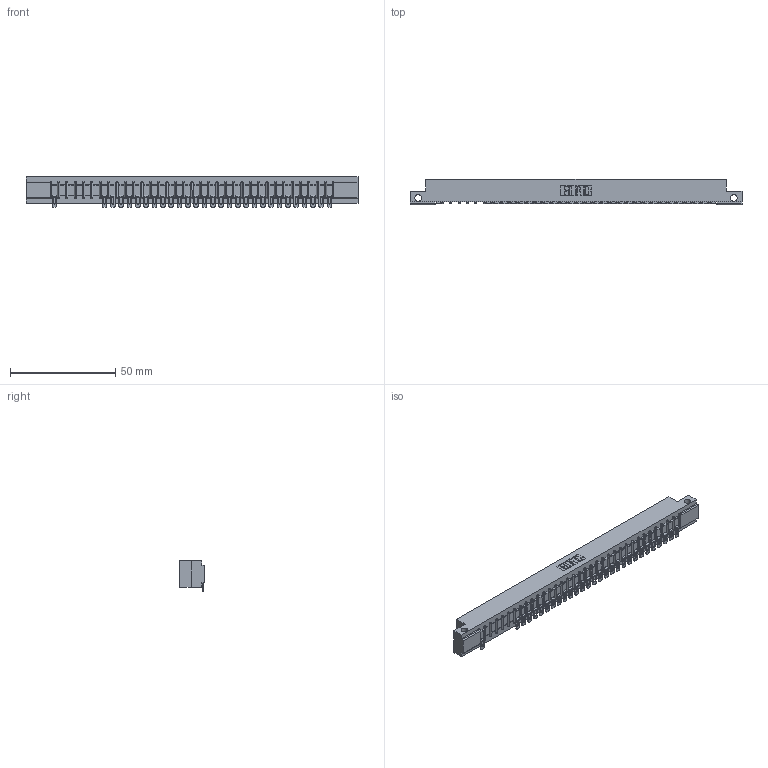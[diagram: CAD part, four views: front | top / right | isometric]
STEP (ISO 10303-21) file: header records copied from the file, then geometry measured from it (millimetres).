
FILE_DESCRIPTION (( 'STEP AP203' ), '1' );
FILE_NAME ('357-034-554-112.STEP', '2018-08-10T02:47:04', ( '' ), ( '' ), 'SwSTEP 2.0', 'SolidWorks 2016', '' );
FILE_SCHEMA (( 'CONFIG_CONTROL_DESIGN' ));
Length unit declared in the file: inch
Products named in the file (3): 307 Part_.128 Dia Side Mounting Holes; 307-290-002_554; 357-034-554-112
Assembly tree (30 placements, depth 2):
  357-034-554-112
    307 Part_.128 Dia Side Mounting Holes
    307-290-002_554  x29
Bounding box: 157.73 x 12.01 x 14.52 mm (x, y, z)
Volume: 16543.5 mm3; surface area: 19800 mm2
Topology: 30 solids, 30 shells, 2602 faces, 7980 edges, 5224 vertices
Faces by surface type: plane 1464, cylinder 1068, sphere 70
Entity records: 30941 total; most frequent: CARTESIAN_POINT 5241, ORIENTED_EDGE 5236, DIRECTION 5096, EDGE_CURVE 2618, LINE 1994, VECTOR 1994, VERTEX_POINT 1696, AXIS2_PLACEMENT_3D 1551
